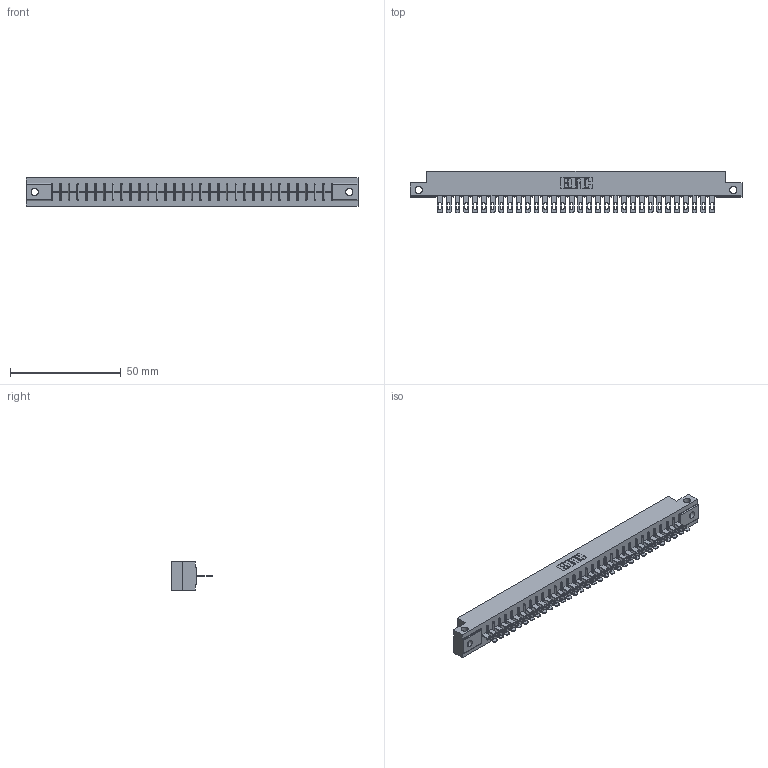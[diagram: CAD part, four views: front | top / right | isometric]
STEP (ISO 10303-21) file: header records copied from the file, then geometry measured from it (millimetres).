
FILE_DESCRIPTION (( 'STEP AP203' ), '1' );
FILE_NAME ('306-032-400-112.STEP', '2020-09-22T02:07:18', ( '' ), ( '' ), 'SwSTEP 2.0', 'SolidWorks 2020', '' );
FILE_SCHEMA (( 'CONFIG_CONTROL_DESIGN' ));
Length unit declared in the file: inch
Products named in the file (3): 306-290-001_100; 306-032-400-112; 306 Part_.128 Dia
Assembly tree (33 placements, depth 2):
  306-032-400-112
    306 Part_.128 Dia
    306-290-001_100  x32
Bounding box: 149.81 x 18.87 x 12.7 mm (x, y, z)
Volume: 16374.8 mm3; surface area: 17301.3 mm2
Topology: 33 solids, 33 shells, 2560 faces, 7232 edges, 4644 vertices
Faces by surface type: plane 1668, cylinder 764, sphere 128
Entity records: 31707 total; most frequent: CARTESIAN_POINT 5371, ORIENTED_EDGE 5280, DIRECTION 5236, EDGE_CURVE 2640, LINE 2042, VECTOR 2042, VERTEX_POINT 1668, AXIS2_PLACEMENT_3D 1597
